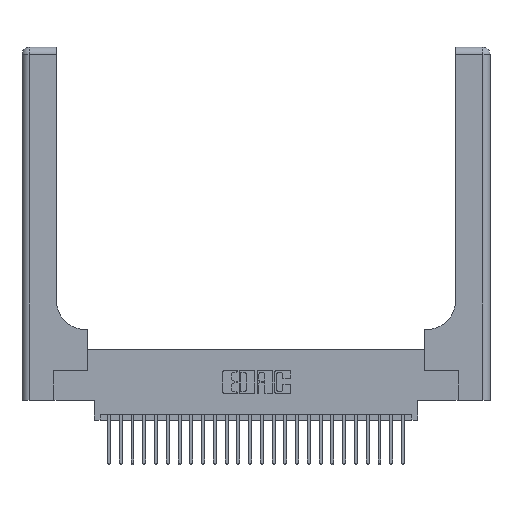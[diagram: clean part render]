
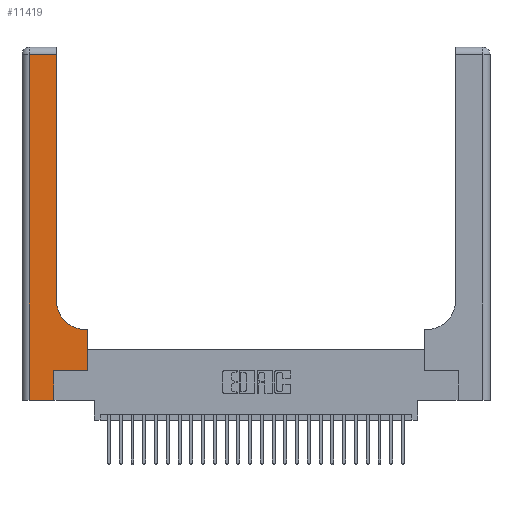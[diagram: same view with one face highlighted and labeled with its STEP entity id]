
A CAD part, top view. The second image highlights one B-rep face of the part: STEP entity #11419.
In plain terms, the highlighted planar face has unit normal (0, 0, 1).
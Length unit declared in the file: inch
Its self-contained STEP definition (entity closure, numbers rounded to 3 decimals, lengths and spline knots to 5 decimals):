
#676 = CARTESIAN_POINT ( 'NONE',  ( 0.269, 0., 0.37 ) ) ;
#909 = LINE ( 'NONE', #2637, #23448 ) ;
#1068 = ORIENTED_EDGE ( 'NONE', *, *, #23983, .T. ) ;
#1333 = ORIENTED_EDGE ( 'NONE', *, *, #9239, .T. ) ;
#1344 = EDGE_LOOP ( 'NONE', ( #1068, #1615, #5413, #18344, #3015, #15700, #1333, #3051, #20955 ) ) ;
#1615 = ORIENTED_EDGE ( 'NONE', *, *, #3803, .T. ) ;
#1843 = CARTESIAN_POINT ( 'NONE',  ( 0.269, 0., 0.37 ) ) ;
#2358 = VECTOR ( 'NONE', #14369, 39.37008 ) ;
#2413 = CARTESIAN_POINT ( 'NONE',  ( 0.2915, 0.85, 0.37 ) ) ;
#2443 = EDGE_CURVE ( 'NONE', #19438, #10451, #20332, .T. ) ;
#2637 = CARTESIAN_POINT ( 'NONE',  ( 0.2915, 3., 0.37 ) ) ;
#3015 = ORIENTED_EDGE ( 'NONE', *, *, #5844, .T. ) ;
#3051 = ORIENTED_EDGE ( 'NONE', *, *, #19283, .T. ) ;
#3351 = CARTESIAN_POINT ( 'NONE',  ( 0.06, 2.94, 0.37 ) ) ;
#3644 = DIRECTION ( 'NONE',  ( 1., 0., 0. ) ) ;
#3803 = EDGE_CURVE ( 'NONE', #17652, #22867, #8267, .T. ) ;
#3830 = CARTESIAN_POINT ( 'NONE',  ( 0.269, 0.25, 0.37 ) ) ;
#3953 = CARTESIAN_POINT ( 'NONE',  ( 0.06, 3., 0.37 ) ) ;
#4304 = LINE ( 'NONE', #9636, #18698 ) ;
#4810 = DIRECTION ( 'NONE',  ( 0., -1., 0. ) ) ;
#5273 = DIRECTION ( 'NONE',  ( 1., 0., 0. ) ) ;
#5413 = ORIENTED_EDGE ( 'NONE', *, *, #15277, .T. ) ;
#5844 = EDGE_CURVE ( 'NONE', #25755, #25991, #17441, .T. ) ;
#7945 = CARTESIAN_POINT ( 'NONE',  ( 0.5415, 0.6, 0.37 ) ) ;
#8267 = LINE ( 'NONE', #12967, #12618 ) ;
#9239 = EDGE_CURVE ( 'NONE', #10459, #21803, #4304, .T. ) ;
#9636 = CARTESIAN_POINT ( 'NONE',  ( 0.5585, 0.25, 0.37 ) ) ;
#9994 = CARTESIAN_POINT ( 'NONE',  ( 0.2915, 0.6, 0.37 ) ) ;
#10331 = VECTOR ( 'NONE', #4810, 39.37008 ) ;
#10451 = VERTEX_POINT ( 'NONE', #2413 ) ;
#10459 = VERTEX_POINT ( 'NONE', #19779 ) ;
#10599 = EDGE_CURVE ( 'NONE', #21702, #25755, #20320, .T. ) ;
#10856 = CARTESIAN_POINT ( 'NONE',  ( 0., 3., 0.37 ) ) ;
#11313 = DIRECTION ( 'NONE',  ( 0., 1., 0. ) ) ;
#11419 = ADVANCED_FACE ( 'NONE', ( #20951 ), #23900, .F. ) ;
#11820 = VECTOR ( 'NONE', #19040, 39.37008 ) ;
#11870 = LINE ( 'NONE', #3830, #21891 ) ;
#12127 = EDGE_CURVE ( 'NONE', #25991, #10459, #11870, .T. ) ;
#12173 = LINE ( 'NONE', #9994, #2358 ) ;
#12303 = VECTOR ( 'NONE', #5273, 39.37008 ) ;
#12618 = VECTOR ( 'NONE', #17411, 39.37008 ) ;
#12967 = CARTESIAN_POINT ( 'NONE',  ( 0., 2.94, 0.37 ) ) ;
#12987 = DIRECTION ( 'NONE',  ( -1., 0., 0. ) ) ;
#14369 = DIRECTION ( 'NONE',  ( -1., 0., 0. ) ) ;
#14423 = CARTESIAN_POINT ( 'NONE',  ( 0.5415, 0.85, 0.37 ) ) ;
#15277 = EDGE_CURVE ( 'NONE', #22867, #21702, #17289, .T. ) ;
#15700 = ORIENTED_EDGE ( 'NONE', *, *, #12127, .T. ) ;
#15854 = AXIS2_PLACEMENT_3D ( 'NONE', #14423, #25260, #18986 ) ;
#16313 = CARTESIAN_POINT ( 'NONE',  ( 0.269, 0.25, 0.37 ) ) ;
#16470 = CARTESIAN_POINT ( 'NONE',  ( 0.2915, 2.94, 0.37 ) ) ;
#17289 = LINE ( 'NONE', #3953, #10331 ) ;
#17411 = DIRECTION ( 'NONE',  ( -1., 0., 0. ) ) ;
#17441 = LINE ( 'NONE', #1843, #11820 ) ;
#17652 = VERTEX_POINT ( 'NONE', #16470 ) ;
#18344 = ORIENTED_EDGE ( 'NONE', *, *, #10599, .T. ) ;
#18585 = CARTESIAN_POINT ( 'NONE',  ( 0.06, 0., 0.37 ) ) ;
#18698 = VECTOR ( 'NONE', #22176, 39.37008 ) ;
#18947 = CARTESIAN_POINT ( 'NONE',  ( 0.5585, 0.6, 0.37 ) ) ;
#18986 = DIRECTION ( 'NONE',  ( 1., 0., 0. ) ) ;
#19040 = DIRECTION ( 'NONE',  ( 0., 1., 0. ) ) ;
#19283 = EDGE_CURVE ( 'NONE', #21803, #19438, #12173, .T. ) ;
#19438 = VERTEX_POINT ( 'NONE', #7945 ) ;
#19779 = CARTESIAN_POINT ( 'NONE',  ( 0.5585, 0.25, 0.37 ) ) ;
#20320 = LINE ( 'NONE', #26533, #12303 ) ;
#20332 = CIRCLE ( 'NONE', #15854, 0.25 ) ;
#20951 = FACE_OUTER_BOUND ( 'NONE', #1344, .T. ) ;
#20955 = ORIENTED_EDGE ( 'NONE', *, *, #2443, .T. ) ;
#21182 = AXIS2_PLACEMENT_3D ( 'NONE', #10856, #25805, #12987 ) ;
#21702 = VERTEX_POINT ( 'NONE', #18585 ) ;
#21803 = VERTEX_POINT ( 'NONE', #18947 ) ;
#21891 = VECTOR ( 'NONE', #3644, 39.37008 ) ;
#22176 = DIRECTION ( 'NONE',  ( 0., 1., 0. ) ) ;
#22867 = VERTEX_POINT ( 'NONE', #3351 ) ;
#23448 = VECTOR ( 'NONE', #11313, 39.37008 ) ;
#23900 = PLANE ( 'NONE',  #21182 ) ;
#23983 = EDGE_CURVE ( 'NONE', #10451, #17652, #909, .T. ) ;
#25260 = DIRECTION ( 'NONE',  ( 0., 0., -1. ) ) ;
#25755 = VERTEX_POINT ( 'NONE', #676 ) ;
#25805 = DIRECTION ( 'NONE',  ( 0., 0., -1. ) ) ;
#25991 = VERTEX_POINT ( 'NONE', #16313 ) ;
#26533 = CARTESIAN_POINT ( 'NONE',  ( 0., 0., 0.37 ) ) ;
